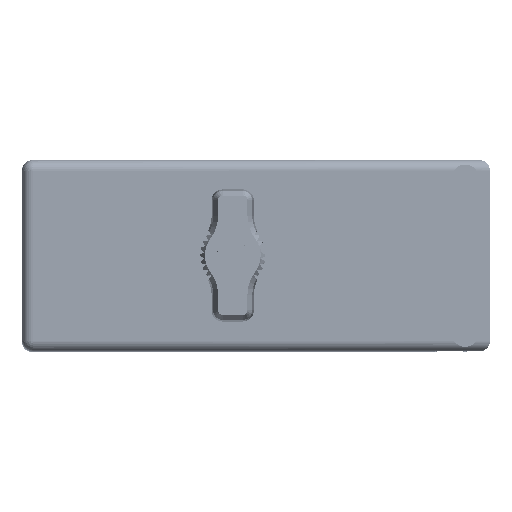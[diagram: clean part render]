
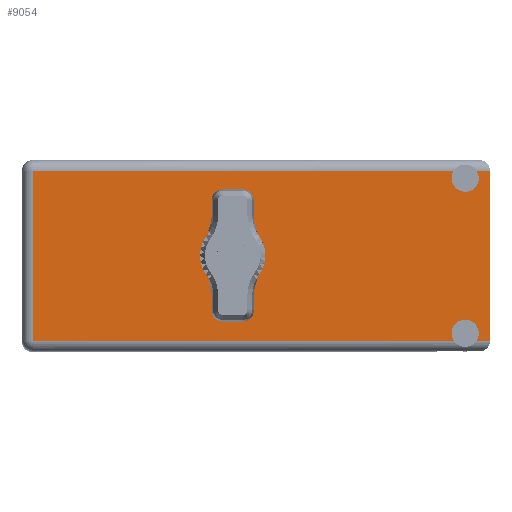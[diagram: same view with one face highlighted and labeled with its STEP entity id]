
A CAD part, top view. The second image highlights one B-rep face of the part: STEP entity #9054.
In plain terms, the highlighted face is planar.
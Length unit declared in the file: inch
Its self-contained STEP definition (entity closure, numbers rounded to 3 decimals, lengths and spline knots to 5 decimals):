
#47 = VERTEX_POINT ( 'NONE', #61228 ) ;
#648 = PLANE ( 'NONE',  #43828 ) ;
#1730 = CARTESIAN_POINT ( 'NONE',  ( 3.018, 1.775, -1.164 ) ) ;
#2512 = CARTESIAN_POINT ( 'NONE',  ( 1.359, 1.775, -0.617 ) ) ;
#2695 = LINE ( 'NONE', #32730, #83475 ) ;
#3043 = CARTESIAN_POINT ( 'NONE',  ( 2.858, 1.775, -0.117 ) ) ;
#5081 = CIRCLE ( 'NONE', #36316, 0.0875 ) ;
#5369 = DIRECTION ( 'NONE',  ( 0., 1., 0. ) ) ;
#6604 = ORIENTED_EDGE ( 'NONE', *, *, #45247, .T. ) ;
#6689 = EDGE_CURVE ( 'NONE', #45188, #49335, #9372, .T. ) ;
#7130 = CARTESIAN_POINT ( 'NONE',  ( 3.018, 1.775, -0.07 ) ) ;
#8159 = VECTOR ( 'NONE', #41387, 39.37008 ) ;
#8795 = DIRECTION ( 'NONE',  ( 0., 1., 0. ) ) ;
#8857 = ORIENTED_EDGE ( 'NONE', *, *, #88153, .T. ) ;
#9054 = ADVANCED_FACE ( 'NONE', ( #81637, #72006 ), #648, .T. ) ;
#9152 = EDGE_CURVE ( 'NONE', #47, #10827, #56860, .T. ) ;
#9372 = CIRCLE ( 'NONE', #50061, 0.125 ) ;
#9691 = CARTESIAN_POINT ( 'NONE',  ( 2.93181, 1.775, -1.164 ) ) ;
#10126 = CARTESIAN_POINT ( 'NONE',  ( 2.78419, 1.775, -1.164 ) ) ;
#10335 = LINE ( 'NONE', #7130, #8159 ) ;
#10827 = VERTEX_POINT ( 'NONE', #60382 ) ;
#11224 = DIRECTION ( 'NONE',  ( 0., 0., 1. ) ) ;
#11230 = CARTESIAN_POINT ( 'NONE',  ( 1.359, 1.775, -0.617 ) ) ;
#12702 = EDGE_LOOP ( 'NONE', ( #79232, #64602 ) ) ;
#16952 = AXIS2_PLACEMENT_3D ( 'NONE', #2512, #71745, #11224 ) ;
#18026 = DIRECTION ( 'NONE',  ( 0., 0., 1. ) ) ;
#19236 = VERTEX_POINT ( 'NONE', #86040 ) ;
#19999 = EDGE_CURVE ( 'NONE', #58120, #78234, #55512, .T. ) ;
#23493 = CARTESIAN_POINT ( 'NONE',  ( 3.018, 1.775, -0.07 ) ) ;
#23637 = ORIENTED_EDGE ( 'NONE', *, *, #9152, .F. ) ;
#25014 = CARTESIAN_POINT ( 'NONE',  ( 2.858, 1.775, -1.117 ) ) ;
#25449 = DIRECTION ( 'NONE',  ( 1., 0., 0. ) ) ;
#25506 = CARTESIAN_POINT ( 'NONE',  ( 2.858, 1.775, -1.117 ) ) ;
#25721 = LINE ( 'NONE', #38450, #41885 ) ;
#26522 = ORIENTED_EDGE ( 'NONE', *, *, #19999, .F. ) ;
#27421 = ORIENTED_EDGE ( 'NONE', *, *, #30040, .T. ) ;
#28621 = VERTEX_POINT ( 'NONE', #29875 ) ;
#29540 = EDGE_CURVE ( 'NONE', #74827, #58120, #5081, .T. ) ;
#29766 = DIRECTION ( 'NONE',  ( 0., 1., 0. ) ) ;
#29875 = CARTESIAN_POINT ( 'NONE',  ( 2.78419, 1.775, -0.07 ) ) ;
#29934 = VECTOR ( 'NONE', #30745, 39.37008 ) ;
#30040 = EDGE_CURVE ( 'NONE', #47, #86467, #10335, .T. ) ;
#30499 = AXIS2_PLACEMENT_3D ( 'NONE', #25014, #39161, #87693 ) ;
#30745 = DIRECTION ( 'NONE',  ( -1., 0., 0. ) ) ;
#31049 = ORIENTED_EDGE ( 'NONE', *, *, #58082, .F. ) ;
#32730 = CARTESIAN_POINT ( 'NONE',  ( 0.07, 1.775, -1.234 ) ) ;
#32859 = EDGE_CURVE ( 'NONE', #19236, #28621, #76496, .T. ) ;
#33293 = DIRECTION ( 'NONE',  ( 0., 0., 1. ) ) ;
#33545 = VECTOR ( 'NONE', #65399, 39.37008 ) ;
#34253 = ORIENTED_EDGE ( 'NONE', *, *, #67284, .T. ) ;
#35539 = DIRECTION ( 'NONE',  ( 0., 0., 1. ) ) ;
#36316 = AXIS2_PLACEMENT_3D ( 'NONE', #25506, #73761, #66811 ) ;
#38450 = CARTESIAN_POINT ( 'NONE',  ( 3.018, 1.775, 0. ) ) ;
#39161 = DIRECTION ( 'NONE',  ( 0., 1., 0. ) ) ;
#39626 = CARTESIAN_POINT ( 'NONE',  ( 2.858, 1.775, -0.117 ) ) ;
#41151 = ORIENTED_EDGE ( 'NONE', *, *, #32859, .T. ) ;
#41387 = DIRECTION ( 'NONE',  ( 1., 0., 0. ) ) ;
#41698 = EDGE_CURVE ( 'NONE', #49335, #45188, #87017, .T. ) ;
#41885 = VECTOR ( 'NONE', #18026, 39.37008 ) ;
#42594 = EDGE_CURVE ( 'NONE', #10827, #28621, #79392, .T. ) ;
#43828 = AXIS2_PLACEMENT_3D ( 'NONE', #69872, #8795, #35539 ) ;
#44610 = DIRECTION ( 'NONE',  ( 0., 1., 0. ) ) ;
#45188 = VERTEX_POINT ( 'NONE', #74315 ) ;
#45247 = EDGE_CURVE ( 'NONE', #47318, #19236, #2695, .T. ) ;
#46344 = EDGE_LOOP ( 'NONE', ( #41151, #76414, #23637, #27421, #31049, #34253, #26522, #63351, #8857, #6604 ) ) ;
#47170 = DIRECTION ( 'NONE',  ( 0., 0., 1. ) ) ;
#47318 = VERTEX_POINT ( 'NONE', #77575 ) ;
#48681 = AXIS2_PLACEMENT_3D ( 'NONE', #39626, #5369, #33293 ) ;
#49335 = VERTEX_POINT ( 'NONE', #86912 ) ;
#50061 = AXIS2_PLACEMENT_3D ( 'NONE', #11230, #44610, #59367 ) ;
#50912 = DIRECTION ( 'NONE',  ( 0., 0., 1. ) ) ;
#50954 = CARTESIAN_POINT ( 'NONE',  ( 0., 1.775, -1.164 ) ) ;
#55090 = LINE ( 'NONE', #50954, #33545 ) ;
#55512 = CIRCLE ( 'NONE', #30499, 0.0875 ) ;
#55712 = VERTEX_POINT ( 'NONE', #1730 ) ;
#56028 = VECTOR ( 'NONE', #25449, 39.37008 ) ;
#56860 = CIRCLE ( 'NONE', #72610, 0.0875 ) ;
#58082 = EDGE_CURVE ( 'NONE', #55712, #86467, #25721, .T. ) ;
#58120 = VERTEX_POINT ( 'NONE', #86965 ) ;
#59367 = DIRECTION ( 'NONE',  ( 0., 0., 1. ) ) ;
#60382 = CARTESIAN_POINT ( 'NONE',  ( 2.858, 1.775, -0.2045 ) ) ;
#61228 = CARTESIAN_POINT ( 'NONE',  ( 2.93181, 1.775, -0.07 ) ) ;
#63351 = ORIENTED_EDGE ( 'NONE', *, *, #29540, .F. ) ;
#64602 = ORIENTED_EDGE ( 'NONE', *, *, #41698, .F. ) ;
#65399 = DIRECTION ( 'NONE',  ( -1., 0., 0. ) ) ;
#66811 = DIRECTION ( 'NONE',  ( 0., 0., 1. ) ) ;
#67284 = EDGE_CURVE ( 'NONE', #55712, #78234, #55090, .T. ) ;
#68750 = LINE ( 'NONE', #78647, #29934 ) ;
#69872 = CARTESIAN_POINT ( 'NONE',  ( 0., 1.775, -1.234 ) ) ;
#71077 = CARTESIAN_POINT ( 'NONE',  ( 3.018, 1.775, -0.07 ) ) ;
#71745 = DIRECTION ( 'NONE',  ( 0., 1., 0. ) ) ;
#72006 = FACE_OUTER_BOUND ( 'NONE', #46344, .T. ) ;
#72610 = AXIS2_PLACEMENT_3D ( 'NONE', #3043, #29766, #50912 ) ;
#73761 = DIRECTION ( 'NONE',  ( 0., 1., 0. ) ) ;
#74315 = CARTESIAN_POINT ( 'NONE',  ( 1.359, 1.775, -0.492 ) ) ;
#74827 = VERTEX_POINT ( 'NONE', #10126 ) ;
#76414 = ORIENTED_EDGE ( 'NONE', *, *, #42594, .F. ) ;
#76496 = LINE ( 'NONE', #23493, #56028 ) ;
#77575 = CARTESIAN_POINT ( 'NONE',  ( 0.07, 1.775, -1.164 ) ) ;
#78234 = VERTEX_POINT ( 'NONE', #9691 ) ;
#78647 = CARTESIAN_POINT ( 'NONE',  ( 0., 1.775, -1.164 ) ) ;
#79232 = ORIENTED_EDGE ( 'NONE', *, *, #6689, .F. ) ;
#79392 = CIRCLE ( 'NONE', #48681, 0.0875 ) ;
#81637 = FACE_BOUND ( 'NONE', #12702, .T. ) ;
#83475 = VECTOR ( 'NONE', #47170, 39.37008 ) ;
#86040 = CARTESIAN_POINT ( 'NONE',  ( 0.07, 1.775, -0.07 ) ) ;
#86467 = VERTEX_POINT ( 'NONE', #71077 ) ;
#86912 = CARTESIAN_POINT ( 'NONE',  ( 1.359, 1.775, -0.742 ) ) ;
#86965 = CARTESIAN_POINT ( 'NONE',  ( 2.858, 1.775, -1.0295 ) ) ;
#87017 = CIRCLE ( 'NONE', #16952, 0.125 ) ;
#87693 = DIRECTION ( 'NONE',  ( 0., 0., 1. ) ) ;
#88153 = EDGE_CURVE ( 'NONE', #74827, #47318, #68750, .T. ) ;
